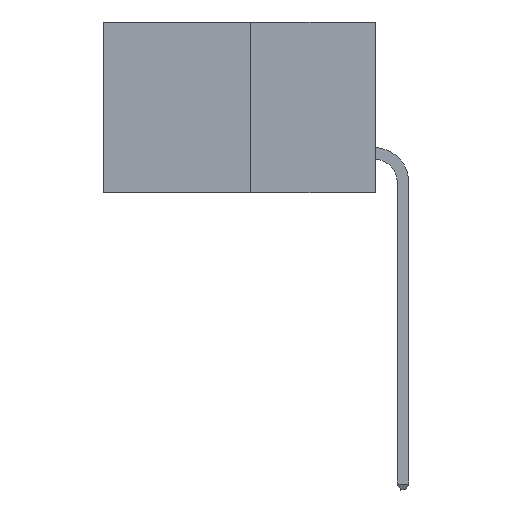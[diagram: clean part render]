
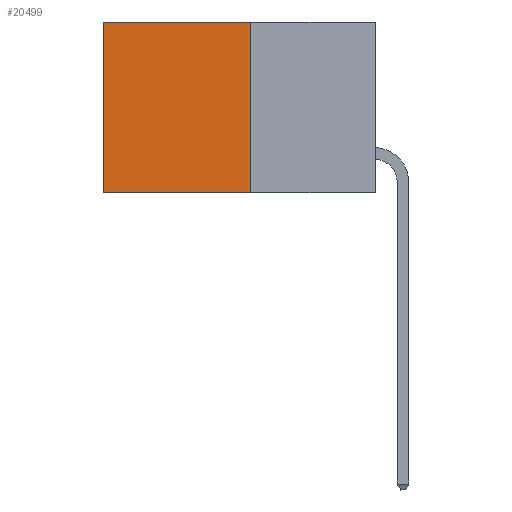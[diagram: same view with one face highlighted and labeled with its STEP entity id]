
A CAD part, left-side view. The second image highlights one B-rep face of the part: STEP entity #20499.
In plain terms, the highlighted planar face has unit normal (-1, 0, 0).
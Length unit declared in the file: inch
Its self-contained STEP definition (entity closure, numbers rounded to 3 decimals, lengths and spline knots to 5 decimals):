
#1639 = DIRECTION ( 'NONE',  ( 0., 1., 0. ) ) ;
#2610 = VERTEX_POINT ( 'NONE', #15011 ) ;
#2756 = VECTOR ( 'NONE', #6996, 39.37008 ) ;
#2762 = VECTOR ( 'NONE', #1639, 39.37008 ) ;
#3319 = VECTOR ( 'NONE', #19481, 39.37008 ) ;
#4162 = CARTESIAN_POINT ( 'NONE',  ( 0.277, 0.27, -0.37 ) ) ;
#4302 = ORIENTED_EDGE ( 'NONE', *, *, #7394, .T. ) ;
#5026 = EDGE_CURVE ( 'NONE', #20671, #17353, #24096, .T. ) ;
#5529 = CARTESIAN_POINT ( 'NONE',  ( 0.277, 0.59, -0.37 ) ) ;
#6996 = DIRECTION ( 'NONE',  ( 0., 0., -1. ) ) ;
#7394 = EDGE_CURVE ( 'NONE', #2610, #14245, #18983, .T. ) ;
#7745 = CARTESIAN_POINT ( 'NONE',  ( 0.277, 0.27, -0.37 ) ) ;
#8960 = CARTESIAN_POINT ( 'NONE',  ( 0.277, 0.59, -0.37 ) ) ;
#9396 = CARTESIAN_POINT ( 'NONE',  ( 0.277, 0.27, -0.37 ) ) ;
#10940 = DIRECTION ( 'NONE',  ( 0., 1., 0. ) ) ;
#11657 = CARTESIAN_POINT ( 'NONE',  ( 0.277, 0.27, -0.37 ) ) ;
#12160 = CARTESIAN_POINT ( 'NONE',  ( 0.277, 0.27, 0. ) ) ;
#12205 = VECTOR ( 'NONE', #10940, 39.37008 ) ;
#12828 = LINE ( 'NONE', #9396, #12205 ) ;
#13378 = CARTESIAN_POINT ( 'NONE',  ( 0.277, 0.27, 0. ) ) ;
#13628 = DIRECTION ( 'NONE',  ( 0., 0., -1. ) ) ;
#13910 = AXIS2_PLACEMENT_3D ( 'NONE', #11657, #25298, #13628 ) ;
#14245 = VERTEX_POINT ( 'NONE', #5529 ) ;
#15011 = CARTESIAN_POINT ( 'NONE',  ( 0.277, 0.59, 0. ) ) ;
#15095 = ORIENTED_EDGE ( 'NONE', *, *, #24920, .F. ) ;
#16503 = ORIENTED_EDGE ( 'NONE', *, *, #5026, .F. ) ;
#17353 = VERTEX_POINT ( 'NONE', #4162 ) ;
#18919 = FACE_OUTER_BOUND ( 'NONE', #22368, .T. ) ;
#18983 = LINE ( 'NONE', #8960, #2756 ) ;
#19455 = PLANE ( 'NONE',  #13910 ) ;
#19481 = DIRECTION ( 'NONE',  ( 0., 0., -1. ) ) ;
#20499 = ADVANCED_FACE ( 'NONE', ( #18919 ), #19455, .F. ) ;
#20671 = VERTEX_POINT ( 'NONE', #12160 ) ;
#22368 = EDGE_LOOP ( 'NONE', ( #4302, #15095, #16503, #22463 ) ) ;
#22463 = ORIENTED_EDGE ( 'NONE', *, *, #24287, .T. ) ;
#22939 = LINE ( 'NONE', #13378, #2762 ) ;
#24096 = LINE ( 'NONE', #7745, #3319 ) ;
#24287 = EDGE_CURVE ( 'NONE', #20671, #2610, #22939, .T. ) ;
#24920 = EDGE_CURVE ( 'NONE', #17353, #14245, #12828, .T. ) ;
#25298 = DIRECTION ( 'NONE',  ( 1., 0., 0. ) ) ;
